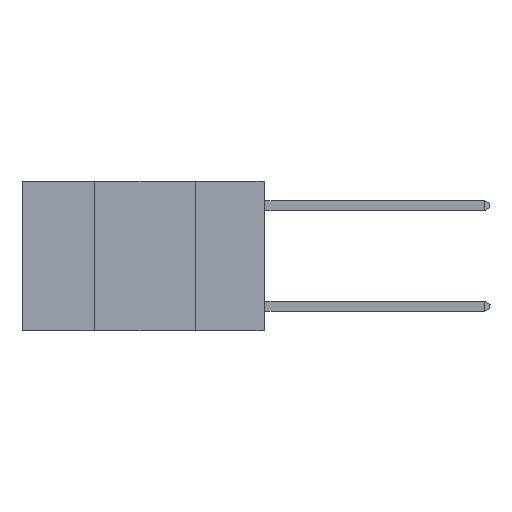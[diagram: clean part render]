
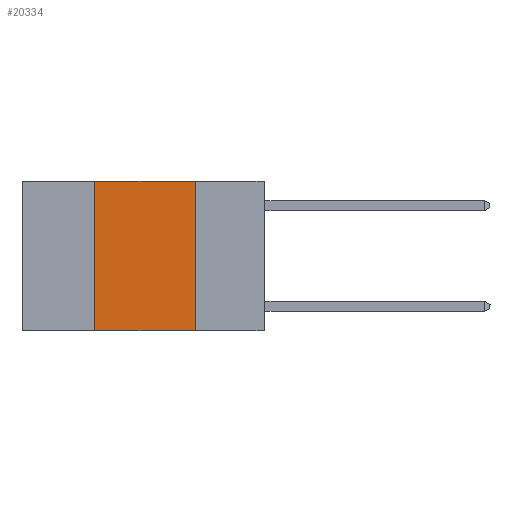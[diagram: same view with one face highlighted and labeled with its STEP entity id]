
A CAD part, left-side view. The second image highlights one B-rep face of the part: STEP entity #20334.
In plain terms, the highlighted planar face has unit normal (-1, 0, 0).
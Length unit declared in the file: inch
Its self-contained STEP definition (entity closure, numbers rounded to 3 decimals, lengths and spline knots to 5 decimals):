
#1141 = VECTOR ( 'NONE', #8417, 39.37008 ) ;
#1332 = CARTESIAN_POINT ( 'NONE',  ( 0., 0.17, 0. ) ) ;
#1900 = VECTOR ( 'NONE', #19907, 39.37008 ) ;
#3661 = EDGE_LOOP ( 'NONE', ( #5827, #10457, #19579, #10988 ) ) ;
#4387 = LINE ( 'NONE', #17674, #17612 ) ;
#4679 = VERTEX_POINT ( 'NONE', #1332 ) ;
#4915 = PLANE ( 'NONE',  #8965 ) ;
#5827 = ORIENTED_EDGE ( 'NONE', *, *, #8562, .F. ) ;
#6403 = LINE ( 'NONE', #22260, #15078 ) ;
#6539 = LINE ( 'NONE', #18199, #1900 ) ;
#7220 = FACE_OUTER_BOUND ( 'NONE', #3661, .T. ) ;
#7259 = CARTESIAN_POINT ( 'NONE',  ( 0., 0.17, -0.37 ) ) ;
#8417 = DIRECTION ( 'NONE',  ( 0., -1., 0. ) ) ;
#8562 = EDGE_CURVE ( 'NONE', #4679, #15432, #6539, .T. ) ;
#8965 = AXIS2_PLACEMENT_3D ( 'NONE', #17051, #10222, #22187 ) ;
#9358 = LINE ( 'NONE', #18760, #1141 ) ;
#10222 = DIRECTION ( 'NONE',  ( 1., 0., 0. ) ) ;
#10457 = ORIENTED_EDGE ( 'NONE', *, *, #17956, .F. ) ;
#10988 = ORIENTED_EDGE ( 'NONE', *, *, #15196, .T. ) ;
#12105 = CARTESIAN_POINT ( 'NONE',  ( 0., 0.42, -0.37 ) ) ;
#12484 = EDGE_CURVE ( 'NONE', #20394, #15476, #6403, .T. ) ;
#15078 = VECTOR ( 'NONE', #20468, 39.37008 ) ;
#15196 = EDGE_CURVE ( 'NONE', #20394, #15432, #9358, .T. ) ;
#15432 = VERTEX_POINT ( 'NONE', #7259 ) ;
#15476 = VERTEX_POINT ( 'NONE', #21101 ) ;
#15942 = DIRECTION ( 'NONE',  ( 0., -1., 0. ) ) ;
#17051 = CARTESIAN_POINT ( 'NONE',  ( 0., 0.6, 0. ) ) ;
#17612 = VECTOR ( 'NONE', #15942, 39.37008 ) ;
#17674 = CARTESIAN_POINT ( 'NONE',  ( 0., 0.6, 0. ) ) ;
#17956 = EDGE_CURVE ( 'NONE', #15476, #4679, #4387, .T. ) ;
#18199 = CARTESIAN_POINT ( 'NONE',  ( 0., 0.17, 0. ) ) ;
#18760 = CARTESIAN_POINT ( 'NONE',  ( 0., 0.6, -0.37 ) ) ;
#19579 = ORIENTED_EDGE ( 'NONE', *, *, #12484, .F. ) ;
#19907 = DIRECTION ( 'NONE',  ( 0., 0., -1. ) ) ;
#20334 = ADVANCED_FACE ( 'NONE', ( #7220 ), #4915, .F. ) ;
#20394 = VERTEX_POINT ( 'NONE', #12105 ) ;
#20468 = DIRECTION ( 'NONE',  ( 0., 0., 1. ) ) ;
#21101 = CARTESIAN_POINT ( 'NONE',  ( 0., 0.42, 0. ) ) ;
#22187 = DIRECTION ( 'NONE',  ( 0., 0., -1. ) ) ;
#22260 = CARTESIAN_POINT ( 'NONE',  ( 0., 0.42, 0. ) ) ;
